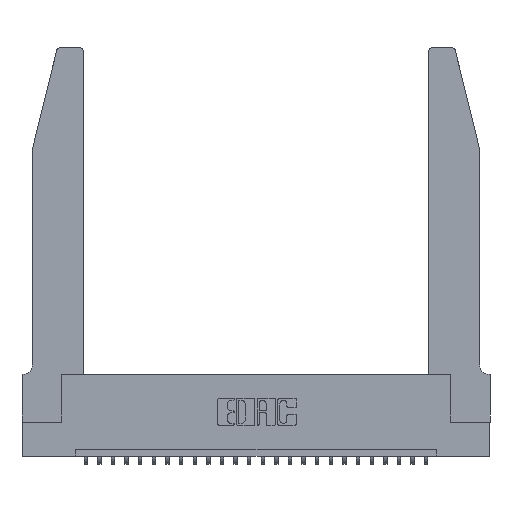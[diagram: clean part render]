
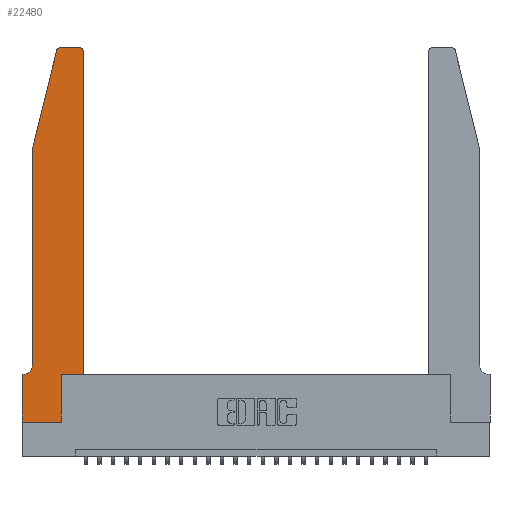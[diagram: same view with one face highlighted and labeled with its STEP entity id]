
A CAD part, top view. The second image highlights one B-rep face of the part: STEP entity #22480.
In plain terms, the highlighted planar face has unit normal (0, 0, 1).
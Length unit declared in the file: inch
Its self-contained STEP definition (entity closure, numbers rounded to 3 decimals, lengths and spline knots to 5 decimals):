
#643 = VECTOR ( 'NONE', #5218, 39.37008 ) ;
#671 = VERTEX_POINT ( 'NONE', #16538 ) ;
#693 = CARTESIAN_POINT ( 'NONE',  ( 0.4505, 0.35, 0.37 ) ) ;
#735 = CARTESIAN_POINT ( 'NONE',  ( 0., 0.35, 0.37 ) ) ;
#980 = CARTESIAN_POINT ( 'NONE',  ( 0., 0.35, 0.37 ) ) ;
#1088 = VECTOR ( 'NONE', #19170, 39.37008 ) ;
#1244 = EDGE_CURVE ( 'NONE', #22749, #8185, #23754, .T. ) ;
#1328 = VECTOR ( 'NONE', #8686, 39.37008 ) ;
#1503 = DIRECTION ( 'NONE',  ( 0., 0., 1. ) ) ;
#1536 = DIRECTION ( 'NONE',  ( -1., 0., 0. ) ) ;
#1596 = ORIENTED_EDGE ( 'NONE', *, *, #4061, .T. ) ;
#1796 = ORIENTED_EDGE ( 'NONE', *, *, #16130, .T. ) ;
#2145 = VECTOR ( 'NONE', #12883, 39.37008 ) ;
#2718 = CARTESIAN_POINT ( 'NONE',  ( 0.4205, 2.72, 0.37 ) ) ;
#2911 = CARTESIAN_POINT ( 'NONE',  ( 0.4505, 0.35, 0.37 ) ) ;
#2962 = VERTEX_POINT ( 'NONE', #21069 ) ;
#2995 = AXIS2_PLACEMENT_3D ( 'NONE', #9933, #3865, #1536 ) ;
#3449 = AXIS2_PLACEMENT_3D ( 'NONE', #13774, #1503, #21660 ) ;
#3865 = DIRECTION ( 'NONE',  ( 0., 0., -1. ) ) ;
#4061 = EDGE_CURVE ( 'NONE', #19342, #8155, #10738, .T. ) ;
#4406 = VERTEX_POINT ( 'NONE', #20402 ) ;
#4536 = ORIENTED_EDGE ( 'NONE', *, *, #15003, .T. ) ;
#4695 = CIRCLE ( 'NONE', #2995, 0.07 ) ;
#4760 = VECTOR ( 'NONE', #10317, 39.37008 ) ;
#5093 = DIRECTION ( 'NONE',  ( 1., 0., 0. ) ) ;
#5106 = ORIENTED_EDGE ( 'NONE', *, *, #20455, .T. ) ;
#5218 = DIRECTION ( 'NONE',  ( -1., 0., 0. ) ) ;
#6697 = EDGE_CURVE ( 'NONE', #21613, #22749, #16379, .T. ) ;
#8116 = VERTEX_POINT ( 'NONE', #735 ) ;
#8155 = VERTEX_POINT ( 'NONE', #8884 ) ;
#8185 = VERTEX_POINT ( 'NONE', #16927 ) ;
#8253 = DIRECTION ( 'NONE',  ( 0., -1., 0. ) ) ;
#8593 = CARTESIAN_POINT ( 'NONE',  ( 0.4505, 0.35, 0.37 ) ) ;
#8595 = ORIENTED_EDGE ( 'NONE', *, *, #6697, .T. ) ;
#8686 = DIRECTION ( 'NONE',  ( -0.239, -0.971, 0. ) ) ;
#8845 = FACE_OUTER_BOUND ( 'NONE', #14733, .T. ) ;
#8884 = CARTESIAN_POINT ( 'NONE',  ( 0.4505, 2.72, 0.37 ) ) ;
#9450 = VECTOR ( 'NONE', #17307, 39.37008 ) ;
#9506 = EDGE_CURVE ( 'NONE', #8116, #2962, #23290, .T. ) ;
#9519 = CARTESIAN_POINT ( 'NONE',  ( 0., 0., 0.37 ) ) ;
#9563 = LINE ( 'NONE', #24509, #4760 ) ;
#9933 = CARTESIAN_POINT ( 'NONE',  ( 0.0055, 0.42, 0.37 ) ) ;
#10083 = ORIENTED_EDGE ( 'NONE', *, *, #18794, .T. ) ;
#10317 = DIRECTION ( 'NONE',  ( -1., 0., 0. ) ) ;
#10663 = LINE ( 'NONE', #693, #1088 ) ;
#10738 = LINE ( 'NONE', #2911, #14299 ) ;
#10933 = DIRECTION ( 'NONE',  ( 1., 0., 0. ) ) ;
#11540 = LINE ( 'NONE', #13276, #643 ) ;
#11876 = VECTOR ( 'NONE', #8253, 39.37008 ) ;
#12183 = CIRCLE ( 'NONE', #23616, 0.03 ) ;
#12883 = DIRECTION ( 'NONE',  ( 0., -1., 0. ) ) ;
#13188 = DIRECTION ( 'NONE',  ( 0., 1., 0. ) ) ;
#13276 = CARTESIAN_POINT ( 'NONE',  ( 0.2605, 2.75, 0.37 ) ) ;
#13475 = DIRECTION ( 'NONE',  ( 0., 1., 0. ) ) ;
#13533 = ORIENTED_EDGE ( 'NONE', *, *, #9506, .T. ) ;
#13774 = CARTESIAN_POINT ( 'NONE',  ( 0.284, 2.72, 0.37 ) ) ;
#13870 = CARTESIAN_POINT ( 'NONE',  ( 0.0755, 2., 0.37 ) ) ;
#14299 = VECTOR ( 'NONE', #13188, 39.37008 ) ;
#14733 = EDGE_LOOP ( 'NONE', ( #17690, #21922, #8595, #15380, #4536, #5106, #13533, #1796, #22860, #18882, #1596, #10083 ) ) ;
#15003 = EDGE_CURVE ( 'NONE', #8185, #16703, #4695, .T. ) ;
#15142 = CARTESIAN_POINT ( 'NONE',  ( 0., 0., 0.37 ) ) ;
#15197 = CIRCLE ( 'NONE', #3449, 0.03 ) ;
#15380 = ORIENTED_EDGE ( 'NONE', *, *, #1244, .T. ) ;
#15982 = CARTESIAN_POINT ( 'NONE',  ( 0.25487, 2.72718, 0.37 ) ) ;
#16074 = EDGE_CURVE ( 'NONE', #16106, #4406, #20992, .T. ) ;
#16106 = VERTEX_POINT ( 'NONE', #21551 ) ;
#16130 = EDGE_CURVE ( 'NONE', #2962, #16106, #26455, .T. ) ;
#16379 = LINE ( 'NONE', #16561, #1328 ) ;
#16397 = CARTESIAN_POINT ( 'NONE',  ( 0.0755, 2., 0.37 ) ) ;
#16538 = CARTESIAN_POINT ( 'NONE',  ( 0.4205, 2.75, 0.37 ) ) ;
#16561 = CARTESIAN_POINT ( 'NONE',  ( 0.0755, 2., 0.37 ) ) ;
#16703 = VERTEX_POINT ( 'NONE', #19656 ) ;
#16927 = CARTESIAN_POINT ( 'NONE',  ( 0.0755, 0.42, 0.37 ) ) ;
#17180 = EDGE_CURVE ( 'NONE', #4406, #19342, #10663, .T. ) ;
#17307 = DIRECTION ( 'NONE',  ( 1., 0., 0. ) ) ;
#17690 = ORIENTED_EDGE ( 'NONE', *, *, #18927, .T. ) ;
#18422 = VECTOR ( 'NONE', #13475, 39.37008 ) ;
#18698 = AXIS2_PLACEMENT_3D ( 'NONE', #980, #25260, #5093 ) ;
#18794 = EDGE_CURVE ( 'NONE', #8155, #671, #12183, .T. ) ;
#18882 = ORIENTED_EDGE ( 'NONE', *, *, #17180, .T. ) ;
#18927 = EDGE_CURVE ( 'NONE', #671, #21270, #11540, .T. ) ;
#19170 = DIRECTION ( 'NONE',  ( 1., 0., 0. ) ) ;
#19342 = VERTEX_POINT ( 'NONE', #8593 ) ;
#19542 = PLANE ( 'NONE',  #18698 ) ;
#19656 = CARTESIAN_POINT ( 'NONE',  ( 0.0055, 0.35, 0.37 ) ) ;
#20402 = CARTESIAN_POINT ( 'NONE',  ( 0.2865, 0.35, 0.37 ) ) ;
#20455 = EDGE_CURVE ( 'NONE', #16703, #8116, #9563, .T. ) ;
#20992 = LINE ( 'NONE', #25760, #18422 ) ;
#21069 = CARTESIAN_POINT ( 'NONE',  ( 0., 0., 0.37 ) ) ;
#21176 = DIRECTION ( 'NONE',  ( 0., 0., 1. ) ) ;
#21270 = VERTEX_POINT ( 'NONE', #23240 ) ;
#21551 = CARTESIAN_POINT ( 'NONE',  ( 0.2865, 0., 0.37 ) ) ;
#21613 = VERTEX_POINT ( 'NONE', #15982 ) ;
#21660 = DIRECTION ( 'NONE',  ( 1., 0., 0. ) ) ;
#21922 = ORIENTED_EDGE ( 'NONE', *, *, #26196, .T. ) ;
#22480 = ADVANCED_FACE ( 'NONE', ( #8845 ), #19542, .T. ) ;
#22749 = VERTEX_POINT ( 'NONE', #13870 ) ;
#22860 = ORIENTED_EDGE ( 'NONE', *, *, #16074, .T. ) ;
#23240 = CARTESIAN_POINT ( 'NONE',  ( 0.284, 2.75, 0.37 ) ) ;
#23290 = LINE ( 'NONE', #15142, #2145 ) ;
#23616 = AXIS2_PLACEMENT_3D ( 'NONE', #2718, #21176, #10933 ) ;
#23754 = LINE ( 'NONE', #16397, #11876 ) ;
#24509 = CARTESIAN_POINT ( 'NONE',  ( 0.0755, 0.35, 0.37 ) ) ;
#25260 = DIRECTION ( 'NONE',  ( 0., 0., 1. ) ) ;
#25760 = CARTESIAN_POINT ( 'NONE',  ( 0.2865, 0.35, 0.37 ) ) ;
#26196 = EDGE_CURVE ( 'NONE', #21270, #21613, #15197, .T. ) ;
#26455 = LINE ( 'NONE', #9519, #9450 ) ;
